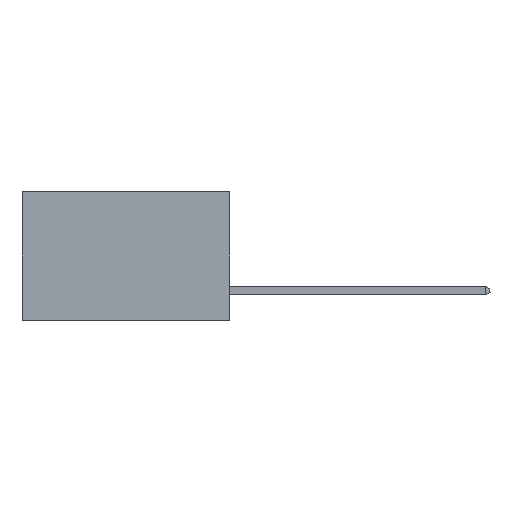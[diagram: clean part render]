
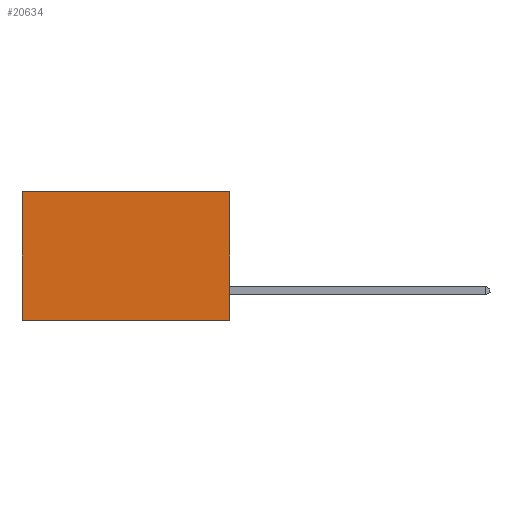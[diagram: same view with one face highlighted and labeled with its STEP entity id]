
A CAD part, left-side view. The second image highlights one B-rep face of the part: STEP entity #20634.
In plain terms, the highlighted planar face has unit normal (-1, 0, 0).
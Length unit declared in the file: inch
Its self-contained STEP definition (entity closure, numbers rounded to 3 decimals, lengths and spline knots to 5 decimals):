
#432 = DIRECTION ( 'NONE',  ( 0., 0., -1. ) ) ;
#1223 = PLANE ( 'NONE',  #11701 ) ;
#1990 = VERTEX_POINT ( 'NONE', #15190 ) ;
#4239 = CARTESIAN_POINT ( 'NONE',  ( 0.298, 0., 0. ) ) ;
#4920 = ORIENTED_EDGE ( 'NONE', *, *, #25710, .T. ) ;
#5798 = CARTESIAN_POINT ( 'NONE',  ( 0.298, 0., 0. ) ) ;
#8421 = FACE_OUTER_BOUND ( 'NONE', #19272, .T. ) ;
#8767 = ORIENTED_EDGE ( 'NONE', *, *, #9929, .F. ) ;
#8773 = DIRECTION ( 'NONE',  ( 0., 1., 0. ) ) ;
#9105 = LINE ( 'NONE', #14786, #12517 ) ;
#9111 = VERTEX_POINT ( 'NONE', #15920 ) ;
#9544 = VECTOR ( 'NONE', #11664, 39.37008 ) ;
#9929 = EDGE_CURVE ( 'NONE', #15453, #1990, #18621, .T. ) ;
#10991 = LINE ( 'NONE', #16254, #20691 ) ;
#11183 = VERTEX_POINT ( 'NONE', #13826 ) ;
#11664 = DIRECTION ( 'NONE',  ( 0., 1., 0. ) ) ;
#11701 = AXIS2_PLACEMENT_3D ( 'NONE', #19147, #23342, #23077 ) ;
#12243 = DIRECTION ( 'NONE',  ( 0., 0., -1. ) ) ;
#12517 = VECTOR ( 'NONE', #8773, 39.37008 ) ;
#12688 = VECTOR ( 'NONE', #12243, 39.37008 ) ;
#13826 = CARTESIAN_POINT ( 'NONE',  ( 0.298, 0.6, 0. ) ) ;
#14250 = LINE ( 'NONE', #5798, #9544 ) ;
#14389 = ORIENTED_EDGE ( 'NONE', *, *, #19946, .F. ) ;
#14786 = CARTESIAN_POINT ( 'NONE',  ( 0.298, 0., -0.37 ) ) ;
#15190 = CARTESIAN_POINT ( 'NONE',  ( 0.298, 0., -0.37 ) ) ;
#15453 = VERTEX_POINT ( 'NONE', #19028 ) ;
#15920 = CARTESIAN_POINT ( 'NONE',  ( 0.298, 0.6, -0.37 ) ) ;
#16254 = CARTESIAN_POINT ( 'NONE',  ( 0.298, 0.6, 0. ) ) ;
#18112 = ORIENTED_EDGE ( 'NONE', *, *, #18612, .T. ) ;
#18612 = EDGE_CURVE ( 'NONE', #11183, #9111, #10991, .T. ) ;
#18621 = LINE ( 'NONE', #4239, #12688 ) ;
#19028 = CARTESIAN_POINT ( 'NONE',  ( 0.298, 0., 0. ) ) ;
#19147 = CARTESIAN_POINT ( 'NONE',  ( 0.298, 0., 0. ) ) ;
#19272 = EDGE_LOOP ( 'NONE', ( #18112, #14389, #8767, #4920 ) ) ;
#19946 = EDGE_CURVE ( 'NONE', #1990, #9111, #9105, .T. ) ;
#20634 = ADVANCED_FACE ( 'NONE', ( #8421 ), #1223, .F. ) ;
#20691 = VECTOR ( 'NONE', #432, 39.37008 ) ;
#23077 = DIRECTION ( 'NONE',  ( 0., 0., -1. ) ) ;
#23342 = DIRECTION ( 'NONE',  ( 1., 0., 0. ) ) ;
#25710 = EDGE_CURVE ( 'NONE', #15453, #11183, #14250, .T. ) ;
